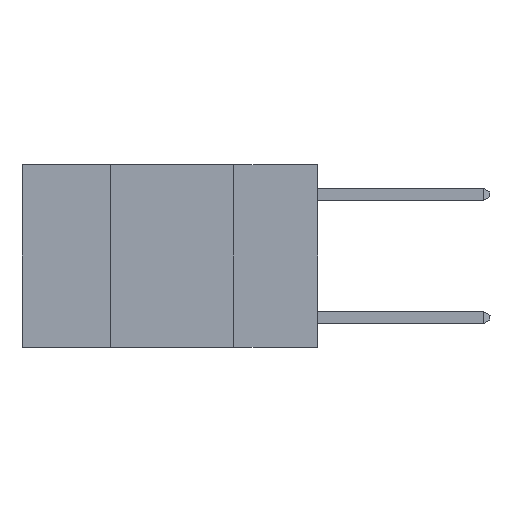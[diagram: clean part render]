
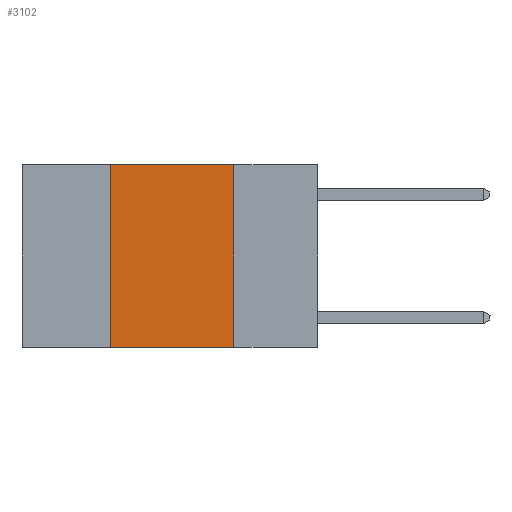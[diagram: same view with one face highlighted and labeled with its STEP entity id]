
A CAD part, left-side view. The second image highlights one B-rep face of the part: STEP entity #3102.
In plain terms, the highlighted planar face has unit normal (-1, 0, 0).
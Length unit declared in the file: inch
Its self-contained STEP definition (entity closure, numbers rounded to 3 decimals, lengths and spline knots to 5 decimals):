
#44 = DIRECTION ( 'NONE',  ( 0., -1., 0. ) ) ;
#397 = VERTEX_POINT ( 'NONE', #5217 ) ;
#1132 = VECTOR ( 'NONE', #16593, 39.37008 ) ;
#1523 = CARTESIAN_POINT ( 'NONE',  ( 0., 0.17, 0. ) ) ;
#2378 = ORIENTED_EDGE ( 'NONE', *, *, #13573, .F. ) ;
#2810 = ORIENTED_EDGE ( 'NONE', *, *, #7965, .F. ) ;
#2897 = CARTESIAN_POINT ( 'NONE',  ( 0., 0.42, 0. ) ) ;
#3102 = ADVANCED_FACE ( 'NONE', ( #13406 ), #3535, .F. ) ;
#3535 = PLANE ( 'NONE',  #9997 ) ;
#3590 = CARTESIAN_POINT ( 'NONE',  ( 0., 0.42, -0.37 ) ) ;
#4100 = CARTESIAN_POINT ( 'NONE',  ( 0., 0.6, 0. ) ) ;
#4698 = VECTOR ( 'NONE', #6424, 39.37008 ) ;
#5138 = VERTEX_POINT ( 'NONE', #1523 ) ;
#5195 = LINE ( 'NONE', #15347, #1132 ) ;
#5217 = CARTESIAN_POINT ( 'NONE',  ( 0., 0.17, -0.37 ) ) ;
#5705 = CARTESIAN_POINT ( 'NONE',  ( 0., 0.42, 0. ) ) ;
#6424 = DIRECTION ( 'NONE',  ( 0., 0., -1. ) ) ;
#6842 = VECTOR ( 'NONE', #6992, 39.37008 ) ;
#6917 = EDGE_CURVE ( 'NONE', #12615, #397, #5195, .T. ) ;
#6923 = EDGE_LOOP ( 'NONE', ( #16500, #2378, #2810, #9971 ) ) ;
#6992 = DIRECTION ( 'NONE',  ( 0., 0., 1. ) ) ;
#7448 = LINE ( 'NONE', #14365, #4698 ) ;
#7965 = EDGE_CURVE ( 'NONE', #12615, #13077, #10372, .T. ) ;
#9028 = EDGE_CURVE ( 'NONE', #5138, #397, #7448, .T. ) ;
#9971 = ORIENTED_EDGE ( 'NONE', *, *, #6917, .T. ) ;
#9997 = AXIS2_PLACEMENT_3D ( 'NONE', #16948, #13328, #12953 ) ;
#10372 = LINE ( 'NONE', #2897, #6842 ) ;
#12615 = VERTEX_POINT ( 'NONE', #3590 ) ;
#12628 = LINE ( 'NONE', #4100, #13479 ) ;
#12953 = DIRECTION ( 'NONE',  ( 0., 0., -1. ) ) ;
#13077 = VERTEX_POINT ( 'NONE', #5705 ) ;
#13328 = DIRECTION ( 'NONE',  ( 1., 0., 0. ) ) ;
#13406 = FACE_OUTER_BOUND ( 'NONE', #6923, .T. ) ;
#13479 = VECTOR ( 'NONE', #44, 39.37008 ) ;
#13573 = EDGE_CURVE ( 'NONE', #13077, #5138, #12628, .T. ) ;
#14365 = CARTESIAN_POINT ( 'NONE',  ( 0., 0.17, 0. ) ) ;
#15347 = CARTESIAN_POINT ( 'NONE',  ( 0., 0.6, -0.37 ) ) ;
#16500 = ORIENTED_EDGE ( 'NONE', *, *, #9028, .F. ) ;
#16593 = DIRECTION ( 'NONE',  ( 0., -1., 0. ) ) ;
#16948 = CARTESIAN_POINT ( 'NONE',  ( 0., 0.6, 0. ) ) ;
